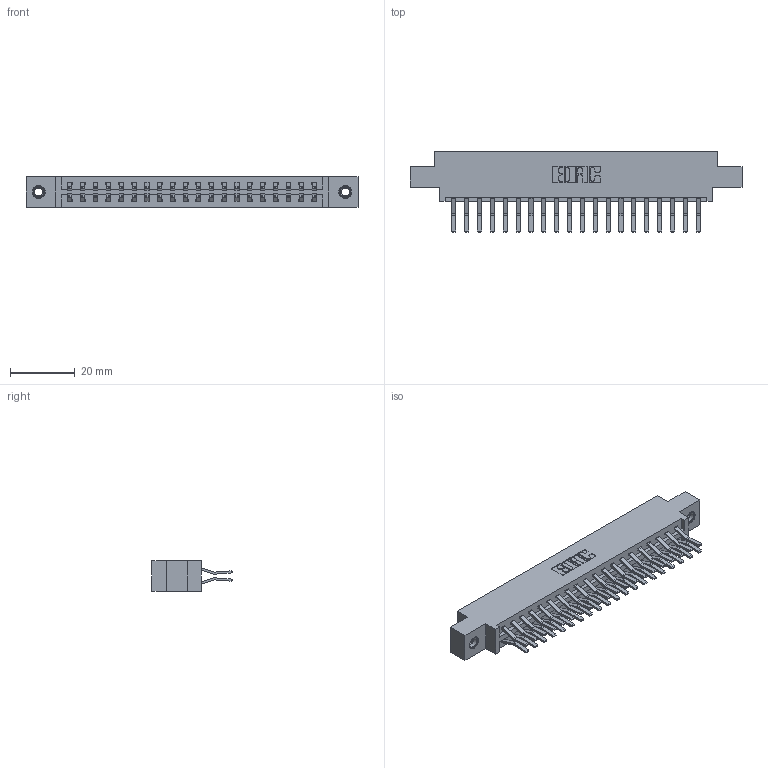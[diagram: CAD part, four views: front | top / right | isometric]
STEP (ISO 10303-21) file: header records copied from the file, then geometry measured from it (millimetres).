
FILE_DESCRIPTION (( 'STEP AP203' ), '1' );
FILE_NAME ('337-040-560-807.STEP', '2018-08-08T21:01:51', ( '' ), ( '' ), 'SwSTEP 2.0', 'SolidWorks 2016', '' );
FILE_SCHEMA (( 'CONFIG_CONTROL_DESIGN' ));
Length unit declared in the file: inch
Products named in the file (4): 337 Part_0.170 Offset - 0.156 Dia-TI; 345-292-001_560 Tail; 345-250-001_345-250-005-103; 337-040-560-807
Assembly tree (43 placements, depth 2):
  337-040-560-807
    337 Part_0.170 Offset - 0.156 Dia-TI
    345-292-001_560 Tail  x40
    345-250-001_345-250-005-103  x2
Bounding box: 102.26 x 24.78 x 9.4 mm (x, y, z)
Volume: 10615.3 mm3; surface area: 12689.6 mm2
Topology: 43 solids, 43 shells, 2418 faces, 7139 edges, 4698 vertices
Faces by surface type: plane 1626, cylinder 776, cone 12, torus 4
Entity records: 19758 total; most frequent: CARTESIAN_POINT 3329, ORIENTED_EDGE 3258, DIRECTION 2907, EDGE_CURVE 1629, LINE 1477, VECTOR 1477, VERTEX_POINT 1080, AXIS2_PLACEMENT_3D 715
